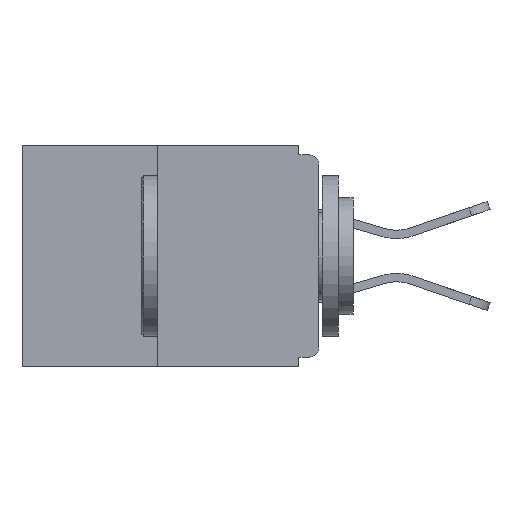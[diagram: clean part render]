
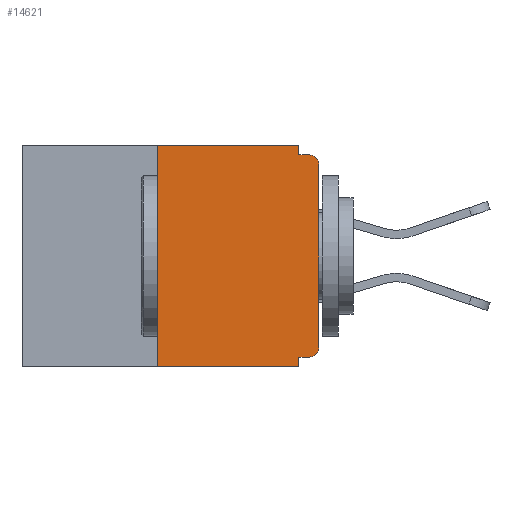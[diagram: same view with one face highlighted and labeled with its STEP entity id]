
A CAD part, left-side view. The second image highlights one B-rep face of the part: STEP entity #14621.
In plain terms, the highlighted planar face has unit normal (-1, 0, 0).
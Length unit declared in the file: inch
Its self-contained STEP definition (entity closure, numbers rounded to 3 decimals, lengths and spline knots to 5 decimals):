
#624 = ORIENTED_EDGE ( 'NONE', *, *, #15109, .F. ) ;
#1006 = VERTEX_POINT ( 'NONE', #5594 ) ;
#1161 = VECTOR ( 'NONE', #16218, 39.37008 ) ;
#1183 = VERTEX_POINT ( 'NONE', #12355 ) ;
#1232 = CARTESIAN_POINT ( 'NONE',  ( 0., 0., -0.015 ) ) ;
#1975 = CARTESIAN_POINT ( 'NONE',  ( 0., 0., -0.313 ) ) ;
#2027 = DIRECTION ( 'NONE',  ( 0., -1., 0. ) ) ;
#2236 = LINE ( 'NONE', #1232, #7531 ) ;
#2363 = VECTOR ( 'NONE', #13013, 39.37008 ) ;
#2526 = ORIENTED_EDGE ( 'NONE', *, *, #6090, .F. ) ;
#2724 = VERTEX_POINT ( 'NONE', #20063 ) ;
#3021 = CARTESIAN_POINT ( 'NONE',  ( 0., 0.031, -0.343 ) ) ;
#3108 = CARTESIAN_POINT ( 'NONE',  ( 0., 0., 0. ) ) ;
#3537 = ORIENTED_EDGE ( 'NONE', *, *, #12417, .T. ) ;
#3543 = DIRECTION ( 'NONE',  ( 0., 0., 1. ) ) ;
#3967 = FACE_OUTER_BOUND ( 'NONE', #5633, .T. ) ;
#4049 = AXIS2_PLACEMENT_3D ( 'NONE', #6158, #7778, #11199 ) ;
#4146 = CARTESIAN_POINT ( 'NONE',  ( 0., 0.25, 0. ) ) ;
#4970 = CARTESIAN_POINT ( 'NONE',  ( 0., 0., -0.328 ) ) ;
#5594 = CARTESIAN_POINT ( 'NONE',  ( 0., 0.25, -0.343 ) ) ;
#5633 = EDGE_LOOP ( 'NONE', ( #2526, #20202, #8524, #18806, #11413, #3537, #12607, #11700, #11607, #624 ) ) ;
#5683 = CARTESIAN_POINT ( 'NONE',  ( 0., 0.46, 0. ) ) ;
#5888 = CARTESIAN_POINT ( 'NONE',  ( 0., 0.031, -0.328 ) ) ;
#6090 = EDGE_CURVE ( 'NONE', #10203, #1183, #15270, .T. ) ;
#6137 = VECTOR ( 'NONE', #3543, 39.37008 ) ;
#6158 = CARTESIAN_POINT ( 'NONE',  ( 0., 0.015, -0.313 ) ) ;
#6423 = CARTESIAN_POINT ( 'NONE',  ( 0., 0.031, 0. ) ) ;
#6488 = DIRECTION ( 'NONE',  ( 0., 0., -1. ) ) ;
#6490 = VECTOR ( 'NONE', #6488, 39.37008 ) ;
#7224 = DIRECTION ( 'NONE',  ( -1., 0., 0. ) ) ;
#7291 = DIRECTION ( 'NONE',  ( 0., 0., -1. ) ) ;
#7531 = VECTOR ( 'NONE', #12731, 39.37008 ) ;
#7778 = DIRECTION ( 'NONE',  ( -1., 0., 0. ) ) ;
#8164 = VERTEX_POINT ( 'NONE', #13555 ) ;
#8524 = ORIENTED_EDGE ( 'NONE', *, *, #18325, .T. ) ;
#8526 = LINE ( 'NONE', #6423, #6490 ) ;
#8607 = CIRCLE ( 'NONE', #4049, 0.015 ) ;
#8722 = LINE ( 'NONE', #4970, #10815 ) ;
#8795 = VERTEX_POINT ( 'NONE', #19719 ) ;
#8904 = VECTOR ( 'NONE', #18220, 39.37008 ) ;
#9151 = VERTEX_POINT ( 'NONE', #5888 ) ;
#9319 = EDGE_CURVE ( 'NONE', #16560, #19012, #2236, .T. ) ;
#9562 = DIRECTION ( 'NONE',  ( 0., 0., -1. ) ) ;
#9800 = LINE ( 'NONE', #3108, #2363 ) ;
#10067 = EDGE_CURVE ( 'NONE', #8795, #9151, #8722, .T. ) ;
#10080 = AXIS2_PLACEMENT_3D ( 'NONE', #5683, #19425, #9562 ) ;
#10203 = VERTEX_POINT ( 'NONE', #4146 ) ;
#10815 = VECTOR ( 'NONE', #16625, 39.37008 ) ;
#10913 = VECTOR ( 'NONE', #2027, 39.37008 ) ;
#11101 = PLANE ( 'NONE',  #10080 ) ;
#11199 = DIRECTION ( 'NONE',  ( 0., 0., -1. ) ) ;
#11413 = ORIENTED_EDGE ( 'NONE', *, *, #10067, .F. ) ;
#11607 = ORIENTED_EDGE ( 'NONE', *, *, #9319, .F. ) ;
#11700 = ORIENTED_EDGE ( 'NONE', *, *, #15972, .T. ) ;
#11727 = CARTESIAN_POINT ( 'NONE',  ( 0., 0.25, 0. ) ) ;
#12355 = CARTESIAN_POINT ( 'NONE',  ( 0., 0.031, 0. ) ) ;
#12417 = EDGE_CURVE ( 'NONE', #8795, #15790, #8607, .T. ) ;
#12607 = ORIENTED_EDGE ( 'NONE', *, *, #16210, .T. ) ;
#12731 = DIRECTION ( 'NONE',  ( 0., -1., 0. ) ) ;
#13013 = DIRECTION ( 'NONE',  ( 0., 0., 1. ) ) ;
#13381 = CARTESIAN_POINT ( 'NONE',  ( 0., 0.015, -0.015 ) ) ;
#13555 = CARTESIAN_POINT ( 'NONE',  ( 0., 0.031, -0.343 ) ) ;
#14621 = ADVANCED_FACE ( 'NONE', ( #3967 ), #11101, .F. ) ;
#14814 = AXIS2_PLACEMENT_3D ( 'NONE', #17034, #7224, #7291 ) ;
#15109 = EDGE_CURVE ( 'NONE', #1183, #16560, #8526, .T. ) ;
#15270 = LINE ( 'NONE', #18588, #10913 ) ;
#15598 = LINE ( 'NONE', #16630, #8904 ) ;
#15790 = VERTEX_POINT ( 'NONE', #1975 ) ;
#15972 = EDGE_CURVE ( 'NONE', #2724, #19012, #20583, .T. ) ;
#16210 = EDGE_CURVE ( 'NONE', #15790, #2724, #9800, .T. ) ;
#16218 = DIRECTION ( 'NONE',  ( 0., 0., -1. ) ) ;
#16560 = VERTEX_POINT ( 'NONE', #20575 ) ;
#16625 = DIRECTION ( 'NONE',  ( 0., 1., 0. ) ) ;
#16630 = CARTESIAN_POINT ( 'NONE',  ( 0., 0.46, -0.343 ) ) ;
#17034 = CARTESIAN_POINT ( 'NONE',  ( 0., 0.015, -0.03 ) ) ;
#17330 = EDGE_CURVE ( 'NONE', #1006, #10203, #20527, .T. ) ;
#17591 = LINE ( 'NONE', #3021, #1161 ) ;
#18220 = DIRECTION ( 'NONE',  ( 0., -1., 0. ) ) ;
#18325 = EDGE_CURVE ( 'NONE', #1006, #8164, #15598, .T. ) ;
#18588 = CARTESIAN_POINT ( 'NONE',  ( 0., 0.46, 0. ) ) ;
#18806 = ORIENTED_EDGE ( 'NONE', *, *, #20506, .F. ) ;
#19012 = VERTEX_POINT ( 'NONE', #13381 ) ;
#19425 = DIRECTION ( 'NONE',  ( 1., 0., 0. ) ) ;
#19719 = CARTESIAN_POINT ( 'NONE',  ( 0., 0.015, -0.328 ) ) ;
#20063 = CARTESIAN_POINT ( 'NONE',  ( 0., 0., -0.03 ) ) ;
#20202 = ORIENTED_EDGE ( 'NONE', *, *, #17330, .F. ) ;
#20506 = EDGE_CURVE ( 'NONE', #9151, #8164, #17591, .T. ) ;
#20527 = LINE ( 'NONE', #11727, #6137 ) ;
#20575 = CARTESIAN_POINT ( 'NONE',  ( 0., 0.031, -0.015 ) ) ;
#20583 = CIRCLE ( 'NONE', #14814, 0.015 ) ;
